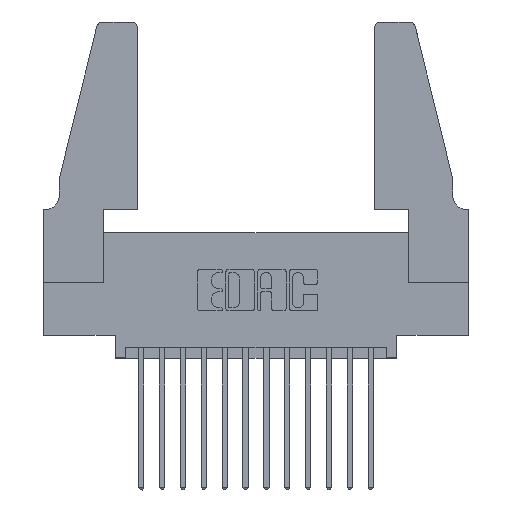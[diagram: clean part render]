
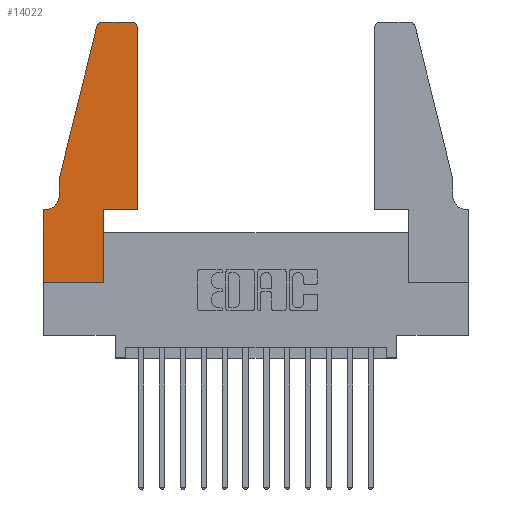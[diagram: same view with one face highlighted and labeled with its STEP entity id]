
A CAD part, top view. The second image highlights one B-rep face of the part: STEP entity #14022.
In plain terms, the highlighted planar face has unit normal (0, 0, 1).
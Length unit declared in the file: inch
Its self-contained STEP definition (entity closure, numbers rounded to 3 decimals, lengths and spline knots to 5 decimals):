
#73 = DIRECTION ( 'NONE',  ( -0.239, -0.971, 0. ) ) ;
#513 = DIRECTION ( 'NONE',  ( 1., 0., 0. ) ) ;
#528 = AXIS2_PLACEMENT_3D ( 'NONE', #13766, #2717, #513 ) ;
#568 = DIRECTION ( 'NONE',  ( 0., 1., 0. ) ) ;
#641 = DIRECTION ( 'NONE',  ( -1., 0., 0. ) ) ;
#734 = LINE ( 'NONE', #15210, #12134 ) ;
#1371 = CIRCLE ( 'NONE', #528, 0.03 ) ;
#1603 = LINE ( 'NONE', #10153, #13787 ) ;
#1717 = EDGE_CURVE ( 'NONE', #13824, #4292, #15677, .T. ) ;
#2099 = EDGE_CURVE ( 'NONE', #13913, #12872, #2733, .T. ) ;
#2717 = DIRECTION ( 'NONE',  ( 0., 0., 1. ) ) ;
#2733 = LINE ( 'NONE', #9508, #7236 ) ;
#2763 = VERTEX_POINT ( 'NONE', #3010 ) ;
#2777 = DIRECTION ( 'NONE',  ( 0., 1., 0. ) ) ;
#2872 = VECTOR ( 'NONE', #5031, 39.37008 ) ;
#3010 = CARTESIAN_POINT ( 'NONE',  ( 0.0755, 0.5, 0.37 ) ) ;
#3231 = VECTOR ( 'NONE', #73, 39.37008 ) ;
#3232 = CARTESIAN_POINT ( 'NONE',  ( 0., 0., 0.37 ) ) ;
#3721 = AXIS2_PLACEMENT_3D ( 'NONE', #11122, #3847, #9150 ) ;
#3847 = DIRECTION ( 'NONE',  ( 0., 0., 1. ) ) ;
#3862 = ORIENTED_EDGE ( 'NONE', *, *, #7384, .T. ) ;
#3986 = ORIENTED_EDGE ( 'NONE', *, *, #9356, .T. ) ;
#4142 = EDGE_CURVE ( 'NONE', #10327, #2763, #14264, .T. ) ;
#4292 = VERTEX_POINT ( 'NONE', #10029 ) ;
#4550 = AXIS2_PLACEMENT_3D ( 'NONE', #11516, #9020, #641 ) ;
#4755 = CARTESIAN_POINT ( 'NONE',  ( 0.2865, 0., 0.37 ) ) ;
#4813 = PLANE ( 'NONE',  #13697 ) ;
#5029 = CARTESIAN_POINT ( 'NONE',  ( 0., 0.35, 0.37 ) ) ;
#5031 = DIRECTION ( 'NONE',  ( 0., -1., 0. ) ) ;
#5071 = EDGE_CURVE ( 'NONE', #7345, #13913, #10978, .T. ) ;
#5190 = ORIENTED_EDGE ( 'NONE', *, *, #2099, .T. ) ;
#5368 = DIRECTION ( 'NONE',  ( -1., 0., 0. ) ) ;
#5494 = CARTESIAN_POINT ( 'NONE',  ( 0.4505, 0.35, 0.37 ) ) ;
#5592 = VERTEX_POINT ( 'NONE', #6861 ) ;
#5895 = DIRECTION ( 'NONE',  ( 0., -1., 0. ) ) ;
#6079 = DIRECTION ( 'NONE',  ( 0., 0., 1. ) ) ;
#6448 = LINE ( 'NONE', #5494, #10257 ) ;
#6618 = CARTESIAN_POINT ( 'NONE',  ( 0., 0.35, 0.37 ) ) ;
#6626 = VECTOR ( 'NONE', #13989, 39.37008 ) ;
#6698 = CARTESIAN_POINT ( 'NONE',  ( 0.4505, 1.22, 0.37 ) ) ;
#6861 = CARTESIAN_POINT ( 'NONE',  ( 0.4505, 0.35, 0.37 ) ) ;
#6987 = ORIENTED_EDGE ( 'NONE', *, *, #7657, .T. ) ;
#7213 = ORIENTED_EDGE ( 'NONE', *, *, #4142, .T. ) ;
#7236 = VECTOR ( 'NONE', #11974, 39.37008 ) ;
#7345 = VERTEX_POINT ( 'NONE', #6618 ) ;
#7384 = EDGE_CURVE ( 'NONE', #7753, #14168, #9386, .T. ) ;
#7657 = EDGE_CURVE ( 'NONE', #12872, #11894, #1603, .T. ) ;
#7753 = VERTEX_POINT ( 'NONE', #10208 ) ;
#7814 = EDGE_CURVE ( 'NONE', #14168, #7345, #14175, .T. ) ;
#8035 = VECTOR ( 'NONE', #13080, 39.37008 ) ;
#8157 = ORIENTED_EDGE ( 'NONE', *, *, #1717, .T. ) ;
#8453 = ORIENTED_EDGE ( 'NONE', *, *, #13137, .T. ) ;
#8463 = ORIENTED_EDGE ( 'NONE', *, *, #7814, .T. ) ;
#8686 = FACE_OUTER_BOUND ( 'NONE', #15113, .T. ) ;
#8798 = CARTESIAN_POINT ( 'NONE',  ( 0.0755, 0.5, 0.37 ) ) ;
#9020 = DIRECTION ( 'NONE',  ( 0., 0., -1. ) ) ;
#9096 = ORIENTED_EDGE ( 'NONE', *, *, #10026, .T. ) ;
#9150 = DIRECTION ( 'NONE',  ( 1., 0., 0. ) ) ;
#9356 = EDGE_CURVE ( 'NONE', #10079, #10327, #1371, .T. ) ;
#9386 = CIRCLE ( 'NONE', #4550, 0.07 ) ;
#9508 = CARTESIAN_POINT ( 'NONE',  ( 0., 0., 0.37 ) ) ;
#9775 = ORIENTED_EDGE ( 'NONE', *, *, #5071, .T. ) ;
#10026 = EDGE_CURVE ( 'NONE', #5592, #13824, #6448, .T. ) ;
#10029 = CARTESIAN_POINT ( 'NONE',  ( 0.4205, 1.25, 0.37 ) ) ;
#10079 = VERTEX_POINT ( 'NONE', #13920 ) ;
#10085 = CARTESIAN_POINT ( 'NONE',  ( 0.2865, 0.35, 0.37 ) ) ;
#10153 = CARTESIAN_POINT ( 'NONE',  ( 0.2865, 0.35, 0.37 ) ) ;
#10208 = CARTESIAN_POINT ( 'NONE',  ( 0.0755, 0.42, 0.37 ) ) ;
#10257 = VECTOR ( 'NONE', #568, 39.37008 ) ;
#10259 = CARTESIAN_POINT ( 'NONE',  ( 0.0755, 0.35, 0.37 ) ) ;
#10327 = VERTEX_POINT ( 'NONE', #11849 ) ;
#10852 = ORIENTED_EDGE ( 'NONE', *, *, #14367, .T. ) ;
#10978 = LINE ( 'NONE', #13282, #13499 ) ;
#11114 = CARTESIAN_POINT ( 'NONE',  ( 0.0055, 0.35, 0.37 ) ) ;
#11122 = CARTESIAN_POINT ( 'NONE',  ( 0.4205, 1.22, 0.37 ) ) ;
#11406 = ORIENTED_EDGE ( 'NONE', *, *, #13052, .T. ) ;
#11516 = CARTESIAN_POINT ( 'NONE',  ( 0.0055, 0.42, 0.37 ) ) ;
#11849 = CARTESIAN_POINT ( 'NONE',  ( 0.25487, 1.22718, 0.37 ) ) ;
#11894 = VERTEX_POINT ( 'NONE', #10085 ) ;
#11974 = DIRECTION ( 'NONE',  ( 1., 0., 0. ) ) ;
#12134 = VECTOR ( 'NONE', #5368, 39.37008 ) ;
#12273 = DIRECTION ( 'NONE',  ( 1., 0., 0. ) ) ;
#12821 = CARTESIAN_POINT ( 'NONE',  ( 0.4505, 0.35, 0.37 ) ) ;
#12872 = VERTEX_POINT ( 'NONE', #4755 ) ;
#13052 = EDGE_CURVE ( 'NONE', #2763, #7753, #13342, .T. ) ;
#13080 = DIRECTION ( 'NONE',  ( -1., 0., 0. ) ) ;
#13137 = EDGE_CURVE ( 'NONE', #11894, #5592, #13894, .T. ) ;
#13282 = CARTESIAN_POINT ( 'NONE',  ( 0., 0., 0.37 ) ) ;
#13342 = LINE ( 'NONE', #8798, #2872 ) ;
#13387 = CARTESIAN_POINT ( 'NONE',  ( 0.0755, 0.5, 0.37 ) ) ;
#13499 = VECTOR ( 'NONE', #5895, 39.37008 ) ;
#13697 = AXIS2_PLACEMENT_3D ( 'NONE', #5029, #6079, #12273 ) ;
#13766 = CARTESIAN_POINT ( 'NONE',  ( 0.284, 1.22, 0.37 ) ) ;
#13787 = VECTOR ( 'NONE', #2777, 39.37008 ) ;
#13824 = VERTEX_POINT ( 'NONE', #6698 ) ;
#13894 = LINE ( 'NONE', #12821, #6626 ) ;
#13913 = VERTEX_POINT ( 'NONE', #3232 ) ;
#13920 = CARTESIAN_POINT ( 'NONE',  ( 0.284, 1.25, 0.37 ) ) ;
#13989 = DIRECTION ( 'NONE',  ( 1., 0., 0. ) ) ;
#14022 = ADVANCED_FACE ( 'NONE', ( #8686 ), #4813, .T. ) ;
#14168 = VERTEX_POINT ( 'NONE', #11114 ) ;
#14175 = LINE ( 'NONE', #10259, #8035 ) ;
#14264 = LINE ( 'NONE', #13387, #3231 ) ;
#14367 = EDGE_CURVE ( 'NONE', #4292, #10079, #734, .T. ) ;
#15113 = EDGE_LOOP ( 'NONE', ( #10852, #3986, #7213, #11406, #3862, #8463, #9775, #5190, #6987, #8453, #9096, #8157 ) ) ;
#15210 = CARTESIAN_POINT ( 'NONE',  ( 0.2605, 1.25, 0.37 ) ) ;
#15677 = CIRCLE ( 'NONE', #3721, 0.03 ) ;
